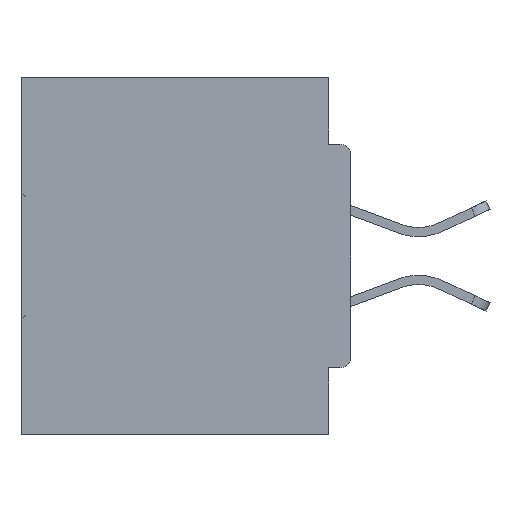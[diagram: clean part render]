
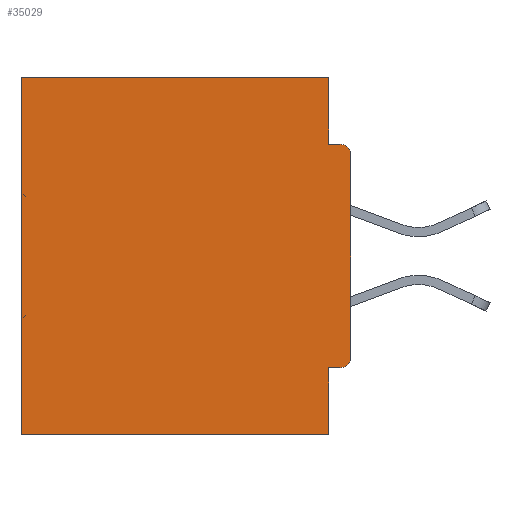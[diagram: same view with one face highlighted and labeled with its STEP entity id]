
A CAD part, left-side view. The second image highlights one B-rep face of the part: STEP entity #35029.
In plain terms, the highlighted planar face has unit normal (-1, 0, 0).
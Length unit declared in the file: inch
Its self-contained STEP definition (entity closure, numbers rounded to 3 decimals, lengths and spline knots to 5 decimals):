
#98 = EDGE_CURVE ( 'NONE', #21287, #9095, #36795, .T. ) ;
#109 = DIRECTION ( 'NONE',  ( 0., 1., 0. ) ) ;
#118 = CARTESIAN_POINT ( 'NONE',  ( 0.298, 0.015, -0.1085 ) ) ;
#442 = VERTEX_POINT ( 'NONE', #30887 ) ;
#1212 = CARTESIAN_POINT ( 'NONE',  ( 0.298, 0., -0.3915 ) ) ;
#1752 = CARTESIAN_POINT ( 'NONE',  ( 0.298, 0.46, 0. ) ) ;
#3856 = EDGE_CURVE ( 'NONE', #20560, #20262, #35806, .T. ) ;
#5306 = EDGE_CURVE ( 'NONE', #20560, #20175, #21059, .T. ) ;
#5819 = ORIENTED_EDGE ( 'NONE', *, *, #5306, .F. ) ;
#7762 = VECTOR ( 'NONE', #109, 39.37008 ) ;
#8165 = CARTESIAN_POINT ( 'NONE',  ( 0.298, 0.015, -0.0935 ) ) ;
#8843 = CARTESIAN_POINT ( 'NONE',  ( 0.298, 0.015, -0.3915 ) ) ;
#9052 = CARTESIAN_POINT ( 'NONE',  ( 0.298, 0.031, 0. ) ) ;
#9095 = VERTEX_POINT ( 'NONE', #16180 ) ;
#9112 = CARTESIAN_POINT ( 'NONE',  ( 0.298, 0.031, -0.0935 ) ) ;
#11259 = CARTESIAN_POINT ( 'NONE',  ( 0.298, 0.031, -0.5 ) ) ;
#11336 = VECTOR ( 'NONE', #23312, 39.37008 ) ;
#13193 = CARTESIAN_POINT ( 'NONE',  ( 0.298, 0.46, 0. ) ) ;
#13520 = DIRECTION ( 'NONE',  ( 0., 0., -1. ) ) ;
#13787 = VERTEX_POINT ( 'NONE', #8165 ) ;
#13843 = CARTESIAN_POINT ( 'NONE',  ( 0.298, 0., -0.1085 ) ) ;
#13853 = CARTESIAN_POINT ( 'NONE',  ( 0.298, 0., 0. ) ) ;
#13965 = CARTESIAN_POINT ( 'NONE',  ( 0.298, 0., 0. ) ) ;
#14200 = EDGE_CURVE ( 'NONE', #20175, #13787, #32832, .T. ) ;
#14450 = ORIENTED_EDGE ( 'NONE', *, *, #38504, .F. ) ;
#14506 = ORIENTED_EDGE ( 'NONE', *, *, #17720, .T. ) ;
#14772 = ORIENTED_EDGE ( 'NONE', *, *, #30579, .T. ) ;
#15229 = VERTEX_POINT ( 'NONE', #45789 ) ;
#16053 = DIRECTION ( 'NONE',  ( -1., 0., 0. ) ) ;
#16055 = LINE ( 'NONE', #13965, #37375 ) ;
#16180 = CARTESIAN_POINT ( 'NONE',  ( 0.298, 0.46, -0.5 ) ) ;
#16199 = DIRECTION ( 'NONE',  ( 0., 0., -1. ) ) ;
#16836 = CARTESIAN_POINT ( 'NONE',  ( 0.298, 0.031, -0.5 ) ) ;
#17720 = EDGE_CURVE ( 'NONE', #20262, #9095, #33274, .T. ) ;
#18063 = DIRECTION ( 'NONE',  ( 0., 1., 0. ) ) ;
#18307 = VECTOR ( 'NONE', #42482, 39.37008 ) ;
#18542 = VECTOR ( 'NONE', #24042, 39.37008 ) ;
#20175 = VERTEX_POINT ( 'NONE', #9112 ) ;
#20262 = VERTEX_POINT ( 'NONE', #13193 ) ;
#20560 = VERTEX_POINT ( 'NONE', #9052 ) ;
#21059 = LINE ( 'NONE', #11259, #35629 ) ;
#21287 = VERTEX_POINT ( 'NONE', #16836 ) ;
#22790 = CARTESIAN_POINT ( 'NONE',  ( 0.298, 0., 0. ) ) ;
#23102 = PLANE ( 'NONE',  #46150 ) ;
#23312 = DIRECTION ( 'NONE',  ( 0., 0., -1. ) ) ;
#24042 = DIRECTION ( 'NONE',  ( 0., 0., -1. ) ) ;
#24954 = DIRECTION ( 'NONE',  ( 0., 0., -1. ) ) ;
#25578 = LINE ( 'NONE', #42330, #18307 ) ;
#26691 = DIRECTION ( 'NONE',  ( 1., 0., 0. ) ) ;
#27422 = ORIENTED_EDGE ( 'NONE', *, *, #14200, .F. ) ;
#28396 = CARTESIAN_POINT ( 'NONE',  ( 0.298, 0., -0.5 ) ) ;
#28825 = DIRECTION ( 'NONE',  ( 0., 0., -1. ) ) ;
#28908 = DIRECTION ( 'NONE',  ( -1., 0., 0. ) ) ;
#29730 = LINE ( 'NONE', #45513, #18542 ) ;
#30579 = EDGE_CURVE ( 'NONE', #41437, #13787, #43520, .T. ) ;
#30887 = CARTESIAN_POINT ( 'NONE',  ( 0.298, 0.015, -0.4065 ) ) ;
#31406 = FACE_OUTER_BOUND ( 'NONE', #32624, .T. ) ;
#32154 = AXIS2_PLACEMENT_3D ( 'NONE', #8843, #16053, #16199 ) ;
#32624 = EDGE_LOOP ( 'NONE', ( #14772, #27422, #5819, #44949, #14506, #43311, #40967, #40141, #44320, #14450 ) ) ;
#32832 = LINE ( 'NONE', #35881, #37846 ) ;
#33274 = LINE ( 'NONE', #1752, #11336 ) ;
#35029 = ADVANCED_FACE ( 'NONE', ( #31406 ), #23102, .F. ) ;
#35629 = VECTOR ( 'NONE', #28825, 39.37008 ) ;
#35806 = LINE ( 'NONE', #13853, #7762 ) ;
#35807 = AXIS2_PLACEMENT_3D ( 'NONE', #118, #28908, #24954 ) ;
#35881 = CARTESIAN_POINT ( 'NONE',  ( 0.298, 0., -0.0935 ) ) ;
#36497 = EDGE_CURVE ( 'NONE', #15229, #21287, #29730, .T. ) ;
#36795 = LINE ( 'NONE', #28396, #38463 ) ;
#37375 = VECTOR ( 'NONE', #13520, 39.37008 ) ;
#37846 = VECTOR ( 'NONE', #39931, 39.37008 ) ;
#38429 = CIRCLE ( 'NONE', #32154, 0.015 ) ;
#38463 = VECTOR ( 'NONE', #18063, 39.37008 ) ;
#38504 = EDGE_CURVE ( 'NONE', #41437, #42497, #16055, .T. ) ;
#38507 = EDGE_CURVE ( 'NONE', #442, #15229, #25578, .T. ) ;
#39931 = DIRECTION ( 'NONE',  ( 0., -1., 0. ) ) ;
#40141 = ORIENTED_EDGE ( 'NONE', *, *, #38507, .F. ) ;
#40938 = DIRECTION ( 'NONE',  ( 0., 0., -1. ) ) ;
#40967 = ORIENTED_EDGE ( 'NONE', *, *, #36497, .F. ) ;
#41437 = VERTEX_POINT ( 'NONE', #13843 ) ;
#42330 = CARTESIAN_POINT ( 'NONE',  ( 0.298, 0., -0.4065 ) ) ;
#42482 = DIRECTION ( 'NONE',  ( 0., 1., 0. ) ) ;
#42497 = VERTEX_POINT ( 'NONE', #1212 ) ;
#43311 = ORIENTED_EDGE ( 'NONE', *, *, #98, .F. ) ;
#43520 = CIRCLE ( 'NONE', #35807, 0.015 ) ;
#44320 = ORIENTED_EDGE ( 'NONE', *, *, #45481, .T. ) ;
#44949 = ORIENTED_EDGE ( 'NONE', *, *, #3856, .T. ) ;
#45481 = EDGE_CURVE ( 'NONE', #442, #42497, #38429, .T. ) ;
#45513 = CARTESIAN_POINT ( 'NONE',  ( 0.298, 0.031, -0.5 ) ) ;
#45789 = CARTESIAN_POINT ( 'NONE',  ( 0.298, 0.031, -0.4065 ) ) ;
#46150 = AXIS2_PLACEMENT_3D ( 'NONE', #22790, #26691, #40938 ) ;
